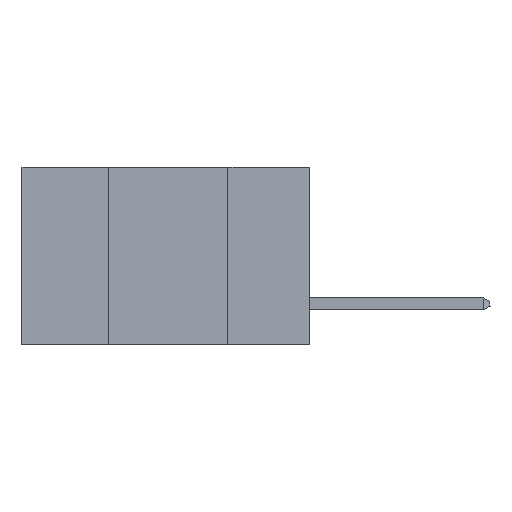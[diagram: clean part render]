
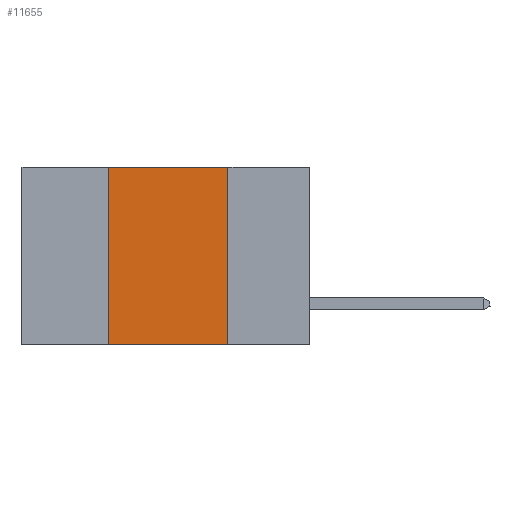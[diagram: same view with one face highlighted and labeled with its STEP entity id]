
A CAD part, left-side view. The second image highlights one B-rep face of the part: STEP entity #11655.
In plain terms, the highlighted planar face has unit normal (-1, 0, 0).
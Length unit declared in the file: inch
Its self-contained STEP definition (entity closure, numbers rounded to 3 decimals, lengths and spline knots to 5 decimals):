
#337 = EDGE_CURVE ( 'NONE', #19130, #3687, #14266, .T. ) ;
#3089 = LINE ( 'NONE', #12460, #8616 ) ;
#3687 = VERTEX_POINT ( 'NONE', #9902 ) ;
#4168 = CARTESIAN_POINT ( 'NONE',  ( 0., 0.17, 0. ) ) ;
#4512 = DIRECTION ( 'NONE',  ( 0., 0., 1. ) ) ;
#4735 = ORIENTED_EDGE ( 'NONE', *, *, #14345, .F. ) ;
#5715 = DIRECTION ( 'NONE',  ( 0., 0., -1. ) ) ;
#6191 = VECTOR ( 'NONE', #16214, 39.37008 ) ;
#7081 = AXIS2_PLACEMENT_3D ( 'NONE', #14704, #7877, #11455 ) ;
#7668 = EDGE_CURVE ( 'NONE', #14402, #3687, #20508, .T. ) ;
#7877 = DIRECTION ( 'NONE',  ( 1., 0., 0. ) ) ;
#7949 = DIRECTION ( 'NONE',  ( 0., -1., 0. ) ) ;
#8135 = EDGE_CURVE ( 'NONE', #14402, #19971, #3089, .T. ) ;
#8616 = VECTOR ( 'NONE', #4512, 39.37008 ) ;
#9608 = CARTESIAN_POINT ( 'NONE',  ( 0., 0.42, -0.37 ) ) ;
#9761 = CARTESIAN_POINT ( 'NONE',  ( 0., 0.6, 0. ) ) ;
#9902 = CARTESIAN_POINT ( 'NONE',  ( 0., 0.17, -0.37 ) ) ;
#11455 = DIRECTION ( 'NONE',  ( 0., 0., -1. ) ) ;
#11655 = ADVANCED_FACE ( 'NONE', ( #12069 ), #18148, .F. ) ;
#12069 = FACE_OUTER_BOUND ( 'NONE', #20291, .T. ) ;
#12460 = CARTESIAN_POINT ( 'NONE',  ( 0., 0.42, 0. ) ) ;
#12980 = ORIENTED_EDGE ( 'NONE', *, *, #7668, .T. ) ;
#14266 = LINE ( 'NONE', #17677, #20300 ) ;
#14321 = CARTESIAN_POINT ( 'NONE',  ( 0., 0.6, -0.37 ) ) ;
#14345 = EDGE_CURVE ( 'NONE', #19971, #19130, #14540, .T. ) ;
#14402 = VERTEX_POINT ( 'NONE', #9608 ) ;
#14540 = LINE ( 'NONE', #9761, #19524 ) ;
#14704 = CARTESIAN_POINT ( 'NONE',  ( 0., 0.6, 0. ) ) ;
#16214 = DIRECTION ( 'NONE',  ( 0., -1., 0. ) ) ;
#17677 = CARTESIAN_POINT ( 'NONE',  ( 0., 0.17, 0. ) ) ;
#18148 = PLANE ( 'NONE',  #7081 ) ;
#18802 = CARTESIAN_POINT ( 'NONE',  ( 0., 0.42, 0. ) ) ;
#19130 = VERTEX_POINT ( 'NONE', #4168 ) ;
#19296 = ORIENTED_EDGE ( 'NONE', *, *, #8135, .F. ) ;
#19524 = VECTOR ( 'NONE', #7949, 39.37008 ) ;
#19971 = VERTEX_POINT ( 'NONE', #18802 ) ;
#20291 = EDGE_LOOP ( 'NONE', ( #21776, #4735, #19296, #12980 ) ) ;
#20300 = VECTOR ( 'NONE', #5715, 39.37008 ) ;
#20508 = LINE ( 'NONE', #14321, #6191 ) ;
#21776 = ORIENTED_EDGE ( 'NONE', *, *, #337, .F. ) ;
